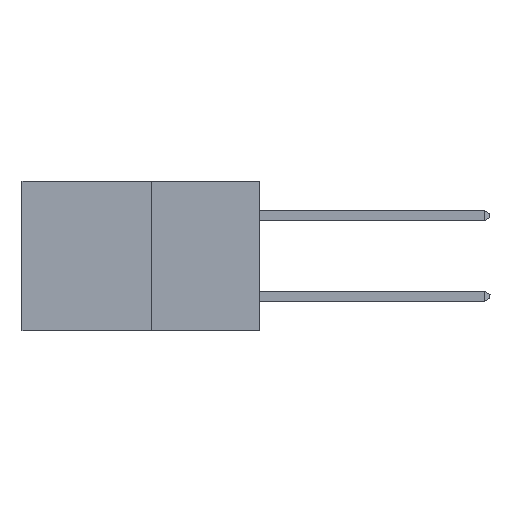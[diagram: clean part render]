
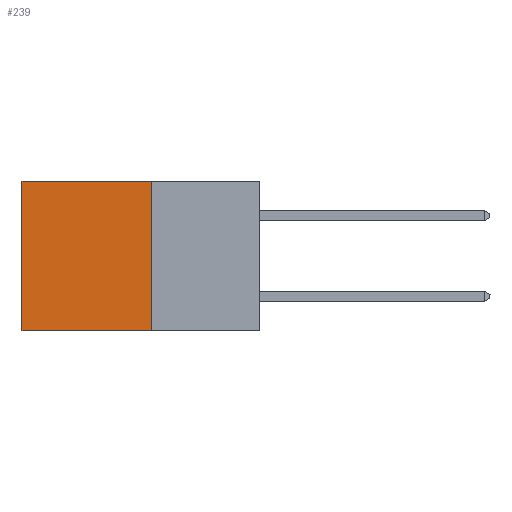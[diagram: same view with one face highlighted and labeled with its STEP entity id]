
A CAD part, left-side view. The second image highlights one B-rep face of the part: STEP entity #239.
In plain terms, the highlighted planar face has unit normal (-1, 0, 0).
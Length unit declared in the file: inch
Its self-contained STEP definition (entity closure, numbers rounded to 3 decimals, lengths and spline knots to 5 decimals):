
#239 = ADVANCED_FACE ( 'NONE', ( #9621 ), #5905, .F. ) ;
#571 = CARTESIAN_POINT ( 'NONE',  ( 0.277, 0.59, -0.37 ) ) ;
#1489 = CARTESIAN_POINT ( 'NONE',  ( 0.277, 0.59, 0. ) ) ;
#1523 = EDGE_CURVE ( 'NONE', #1977, #2745, #2835, .T. ) ;
#1798 = ORIENTED_EDGE ( 'NONE', *, *, #10918, .T. ) ;
#1977 = VERTEX_POINT ( 'NONE', #5602 ) ;
#2148 = DIRECTION ( 'NONE',  ( 0., 0., -1. ) ) ;
#2745 = VERTEX_POINT ( 'NONE', #3955 ) ;
#2835 = LINE ( 'NONE', #3311, #7312 ) ;
#3311 = CARTESIAN_POINT ( 'NONE',  ( 0.277, 0.27, -0.37 ) ) ;
#3442 = CARTESIAN_POINT ( 'NONE',  ( 0.277, 0.27, -0.37 ) ) ;
#3743 = VECTOR ( 'NONE', #4911, 39.37008 ) ;
#3955 = CARTESIAN_POINT ( 'NONE',  ( 0.277, 0.27, -0.37 ) ) ;
#4384 = ORIENTED_EDGE ( 'NONE', *, *, #1523, .F. ) ;
#4621 = AXIS2_PLACEMENT_3D ( 'NONE', #3442, #5606, #2148 ) ;
#4778 = CARTESIAN_POINT ( 'NONE',  ( 0.277, 0.27, -0.37 ) ) ;
#4788 = CARTESIAN_POINT ( 'NONE',  ( 0.277, 0.59, -0.37 ) ) ;
#4850 = ORIENTED_EDGE ( 'NONE', *, *, #10534, .F. ) ;
#4911 = DIRECTION ( 'NONE',  ( 0., 0., -1. ) ) ;
#4920 = CARTESIAN_POINT ( 'NONE',  ( 0.277, 0.27, 0. ) ) ;
#5019 = DIRECTION ( 'NONE',  ( 0., 1., 0. ) ) ;
#5572 = EDGE_CURVE ( 'NONE', #1977, #5793, #11020, .T. ) ;
#5600 = DIRECTION ( 'NONE',  ( 0., 1., 0. ) ) ;
#5602 = CARTESIAN_POINT ( 'NONE',  ( 0.277, 0.27, 0. ) ) ;
#5606 = DIRECTION ( 'NONE',  ( 1., 0., 0. ) ) ;
#5721 = EDGE_LOOP ( 'NONE', ( #1798, #4850, #4384, #7426 ) ) ;
#5732 = LINE ( 'NONE', #571, #3743 ) ;
#5793 = VERTEX_POINT ( 'NONE', #1489 ) ;
#5905 = PLANE ( 'NONE',  #4621 ) ;
#6466 = DIRECTION ( 'NONE',  ( 0., 0., -1. ) ) ;
#6764 = VECTOR ( 'NONE', #5019, 39.37008 ) ;
#6928 = VECTOR ( 'NONE', #5600, 39.37008 ) ;
#7183 = LINE ( 'NONE', #4778, #6928 ) ;
#7312 = VECTOR ( 'NONE', #6466, 39.37008 ) ;
#7426 = ORIENTED_EDGE ( 'NONE', *, *, #5572, .T. ) ;
#9621 = FACE_OUTER_BOUND ( 'NONE', #5721, .T. ) ;
#9820 = VERTEX_POINT ( 'NONE', #4788 ) ;
#10534 = EDGE_CURVE ( 'NONE', #2745, #9820, #7183, .T. ) ;
#10918 = EDGE_CURVE ( 'NONE', #5793, #9820, #5732, .T. ) ;
#11020 = LINE ( 'NONE', #4920, #6764 ) ;
